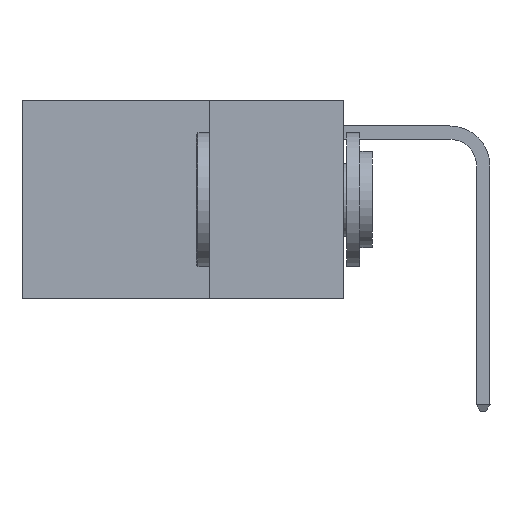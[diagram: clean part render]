
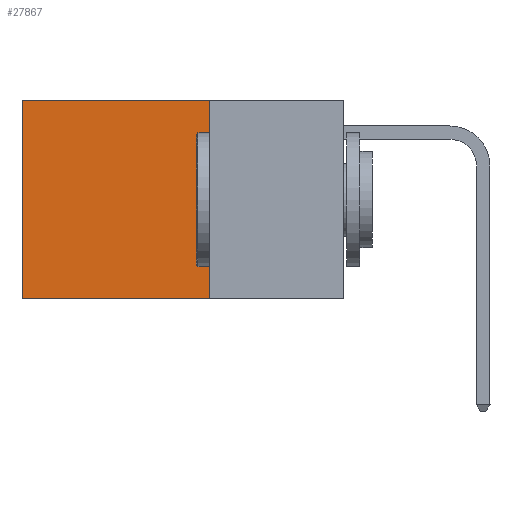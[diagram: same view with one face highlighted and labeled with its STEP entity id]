
A CAD part, left-side view. The second image highlights one B-rep face of the part: STEP entity #27867.
In plain terms, the highlighted planar face has unit normal (-1, 0, 0).
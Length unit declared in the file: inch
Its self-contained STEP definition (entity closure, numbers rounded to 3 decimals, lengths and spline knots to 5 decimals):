
#598 = VECTOR ( 'NONE', #4383, 39.37008 ) ;
#783 = DIRECTION ( 'NONE',  ( 1., 0., 0. ) ) ;
#1275 = AXIS2_PLACEMENT_3D ( 'NONE', #15635, #783, #3301 ) ;
#2193 = VERTEX_POINT ( 'NONE', #18083 ) ;
#3301 = DIRECTION ( 'NONE',  ( 0., 0., -1. ) ) ;
#4383 = DIRECTION ( 'NONE',  ( 0., 0., -1. ) ) ;
#4536 = CARTESIAN_POINT ( 'NONE',  ( 0.2625, 0.25, 0. ) ) ;
#4735 = LINE ( 'NONE', #26450, #27485 ) ;
#5243 = VERTEX_POINT ( 'NONE', #14929 ) ;
#5521 = FACE_OUTER_BOUND ( 'NONE', #25159, .T. ) ;
#5716 = LINE ( 'NONE', #18000, #24351 ) ;
#6396 = EDGE_CURVE ( 'NONE', #27443, #2193, #12115, .T. ) ;
#10356 = DIRECTION ( 'NONE',  ( 0., 1., 0. ) ) ;
#10411 = ORIENTED_EDGE ( 'NONE', *, *, #6396, .F. ) ;
#11607 = ORIENTED_EDGE ( 'NONE', *, *, #12868, .T. ) ;
#12115 = LINE ( 'NONE', #4536, #598 ) ;
#12804 = PLANE ( 'NONE',  #1275 ) ;
#12868 = EDGE_CURVE ( 'NONE', #27443, #27199, #22305, .T. ) ;
#13155 = DIRECTION ( 'NONE',  ( 0., 0., -1. ) ) ;
#14929 = CARTESIAN_POINT ( 'NONE',  ( 0.2625, 0.6, -0.37 ) ) ;
#15374 = EDGE_CURVE ( 'NONE', #2193, #5243, #4735, .T. ) ;
#15635 = CARTESIAN_POINT ( 'NONE',  ( 0.2625, 0.25, 0. ) ) ;
#16958 = VECTOR ( 'NONE', #10356, 39.37008 ) ;
#18000 = CARTESIAN_POINT ( 'NONE',  ( 0.2625, 0.6, 0. ) ) ;
#18083 = CARTESIAN_POINT ( 'NONE',  ( 0.2625, 0.25, -0.37 ) ) ;
#20258 = CARTESIAN_POINT ( 'NONE',  ( 0.2625, 0.25, 0. ) ) ;
#22305 = LINE ( 'NONE', #20258, #16958 ) ;
#23625 = DIRECTION ( 'NONE',  ( 0., 1., 0. ) ) ;
#24351 = VECTOR ( 'NONE', #13155, 39.37008 ) ;
#25067 = CARTESIAN_POINT ( 'NONE',  ( 0.2625, 0.25, 0. ) ) ;
#25159 = EDGE_LOOP ( 'NONE', ( #27982, #26126, #10411, #11607 ) ) ;
#26070 = CARTESIAN_POINT ( 'NONE',  ( 0.2625, 0.6, 0. ) ) ;
#26080 = EDGE_CURVE ( 'NONE', #27199, #5243, #5716, .T. ) ;
#26126 = ORIENTED_EDGE ( 'NONE', *, *, #15374, .F. ) ;
#26450 = CARTESIAN_POINT ( 'NONE',  ( 0.2625, 0.25, -0.37 ) ) ;
#27199 = VERTEX_POINT ( 'NONE', #26070 ) ;
#27443 = VERTEX_POINT ( 'NONE', #25067 ) ;
#27485 = VECTOR ( 'NONE', #23625, 39.37008 ) ;
#27867 = ADVANCED_FACE ( 'NONE', ( #5521 ), #12804, .F. ) ;
#27982 = ORIENTED_EDGE ( 'NONE', *, *, #26080, .T. ) ;
